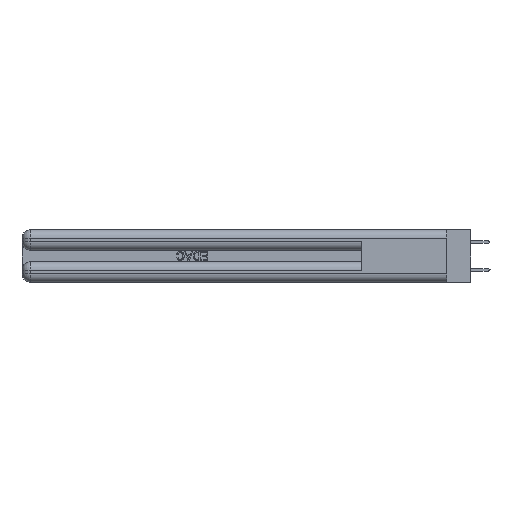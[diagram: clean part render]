
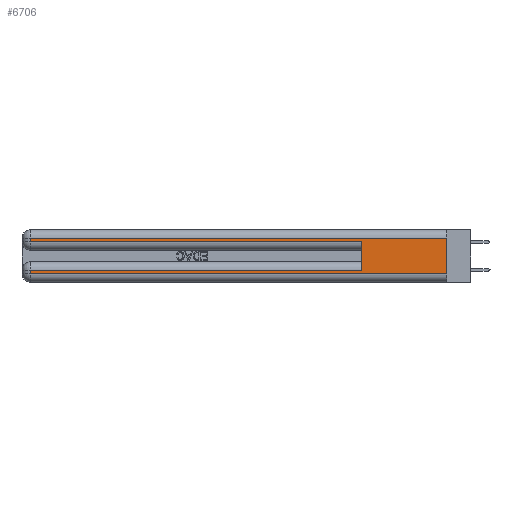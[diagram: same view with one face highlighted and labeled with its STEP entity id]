
A CAD part, left-side view. The second image highlights one B-rep face of the part: STEP entity #6706.
In plain terms, the highlighted planar face has unit normal (-1, 0, 0).
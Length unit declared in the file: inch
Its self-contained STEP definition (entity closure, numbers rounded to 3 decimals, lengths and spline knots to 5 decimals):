
#195 = DIRECTION ( 'NONE',  ( 0., 0., -1. ) ) ;
#430 = CARTESIAN_POINT ( 'NONE',  ( 0., 0.6, 0.085 ) ) ;
#1336 = EDGE_CURVE ( 'NONE', #7126, #42775, #39232, .T. ) ;
#2205 = VECTOR ( 'NONE', #15513, 39.37008 ) ;
#2762 = VERTEX_POINT ( 'NONE', #13270 ) ;
#4721 = EDGE_CURVE ( 'NONE', #42775, #9584, #18332, .T. ) ;
#4777 = VECTOR ( 'NONE', #13928, 39.37008 ) ;
#4791 = DIRECTION ( 'NONE',  ( 1., 0., 0. ) ) ;
#6706 = ADVANCED_FACE ( 'NONE', ( #21911 ), #29560, .F. ) ;
#7126 = VERTEX_POINT ( 'NONE', #13846 ) ;
#7236 = CARTESIAN_POINT ( 'NONE',  ( 0., 2.94, 0.37 ) ) ;
#7890 = DIRECTION ( 'NONE',  ( 0., 1., 0. ) ) ;
#7970 = CARTESIAN_POINT ( 'NONE',  ( 0., 0.6, 0.145 ) ) ;
#8165 = VECTOR ( 'NONE', #7890, 39.37008 ) ;
#8283 = EDGE_CURVE ( 'NONE', #30351, #14307, #21940, .T. ) ;
#8324 = VECTOR ( 'NONE', #44380, 39.37008 ) ;
#9584 = VERTEX_POINT ( 'NONE', #42636 ) ;
#10337 = VECTOR ( 'NONE', #43125, 39.37008 ) ;
#10439 = CARTESIAN_POINT ( 'NONE',  ( 0., 2.94, 0.06 ) ) ;
#10792 = ORIENTED_EDGE ( 'NONE', *, *, #32979, .F. ) ;
#11265 = CARTESIAN_POINT ( 'NONE',  ( 0., 2.94, 0.31 ) ) ;
#11811 = CARTESIAN_POINT ( 'NONE',  ( 0., 2.94, 0.37 ) ) ;
#12720 = CARTESIAN_POINT ( 'NONE',  ( 0., 0., 0.285 ) ) ;
#12822 = EDGE_CURVE ( 'NONE', #17526, #21117, #39930, .T. ) ;
#13270 = CARTESIAN_POINT ( 'NONE',  ( 0., 2.94, 0.285 ) ) ;
#13846 = CARTESIAN_POINT ( 'NONE',  ( 0., 2.94, 0.085 ) ) ;
#13928 = DIRECTION ( 'NONE',  ( 0., 0., -1. ) ) ;
#14121 = DIRECTION ( 'NONE',  ( 0., -1., 0. ) ) ;
#14307 = VERTEX_POINT ( 'NONE', #11265 ) ;
#14349 = ORIENTED_EDGE ( 'NONE', *, *, #12822, .F. ) ;
#14355 = EDGE_LOOP ( 'NONE', ( #10792, #32891, #43515, #46028, #14349, #40046, #27246, #40317 ) ) ;
#14660 = LINE ( 'NONE', #11811, #10337 ) ;
#15513 = DIRECTION ( 'NONE',  ( 0., 1., 0. ) ) ;
#17526 = VERTEX_POINT ( 'NONE', #430 ) ;
#18332 = LINE ( 'NONE', #32559, #33151 ) ;
#19784 = LINE ( 'NONE', #12720, #24498 ) ;
#20225 = VECTOR ( 'NONE', #195, 39.37008 ) ;
#21117 = VERTEX_POINT ( 'NONE', #31944 ) ;
#21911 = FACE_OUTER_BOUND ( 'NONE', #14355, .T. ) ;
#21940 = LINE ( 'NONE', #32641, #8165 ) ;
#22008 = CARTESIAN_POINT ( 'NONE',  ( 0., 0., 0.31 ) ) ;
#24498 = VECTOR ( 'NONE', #26535, 39.37008 ) ;
#26535 = DIRECTION ( 'NONE',  ( 0., -1., 0. ) ) ;
#27246 = ORIENTED_EDGE ( 'NONE', *, *, #1336, .T. ) ;
#27706 = LINE ( 'NONE', #42388, #4777 ) ;
#29512 = CARTESIAN_POINT ( 'NONE',  ( 0., 0., 0.085 ) ) ;
#29560 = PLANE ( 'NONE',  #43130 ) ;
#29783 = CARTESIAN_POINT ( 'NONE',  ( 0., 0., 0.37 ) ) ;
#30351 = VERTEX_POINT ( 'NONE', #22008 ) ;
#31944 = CARTESIAN_POINT ( 'NONE',  ( 0., 0.6, 0.285 ) ) ;
#32559 = CARTESIAN_POINT ( 'NONE',  ( 0., 0., 0.06 ) ) ;
#32572 = LINE ( 'NONE', #29512, #2205 ) ;
#32641 = CARTESIAN_POINT ( 'NONE',  ( 0., 0., 0.31 ) ) ;
#32891 = ORIENTED_EDGE ( 'NONE', *, *, #8283, .T. ) ;
#32979 = EDGE_CURVE ( 'NONE', #30351, #9584, #27706, .T. ) ;
#33151 = VECTOR ( 'NONE', #14121, 39.37008 ) ;
#36112 = DIRECTION ( 'NONE',  ( 0., 0., -1. ) ) ;
#39232 = LINE ( 'NONE', #7236, #20225 ) ;
#39930 = LINE ( 'NONE', #7970, #8324 ) ;
#40046 = ORIENTED_EDGE ( 'NONE', *, *, #43149, .T. ) ;
#40317 = ORIENTED_EDGE ( 'NONE', *, *, #4721, .T. ) ;
#40595 = EDGE_CURVE ( 'NONE', #2762, #21117, #19784, .T. ) ;
#41651 = EDGE_CURVE ( 'NONE', #14307, #2762, #14660, .T. ) ;
#42388 = CARTESIAN_POINT ( 'NONE',  ( 0., 0., 0.37 ) ) ;
#42636 = CARTESIAN_POINT ( 'NONE',  ( 0., 0., 0.06 ) ) ;
#42775 = VERTEX_POINT ( 'NONE', #10439 ) ;
#43125 = DIRECTION ( 'NONE',  ( 0., 0., -1. ) ) ;
#43130 = AXIS2_PLACEMENT_3D ( 'NONE', #29783, #4791, #36112 ) ;
#43149 = EDGE_CURVE ( 'NONE', #17526, #7126, #32572, .T. ) ;
#43515 = ORIENTED_EDGE ( 'NONE', *, *, #41651, .T. ) ;
#44380 = DIRECTION ( 'NONE',  ( 0., 0., 1. ) ) ;
#46028 = ORIENTED_EDGE ( 'NONE', *, *, #40595, .T. ) ;
